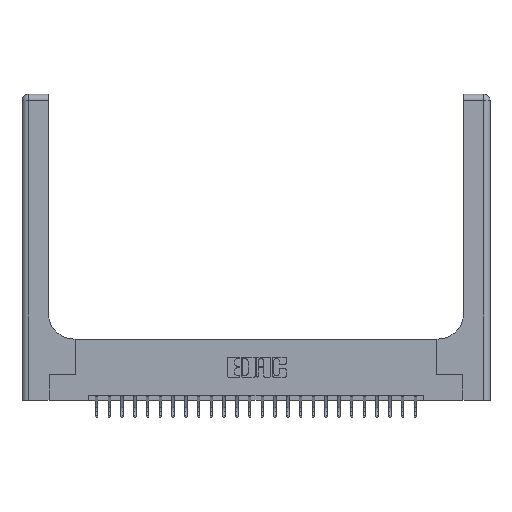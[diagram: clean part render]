
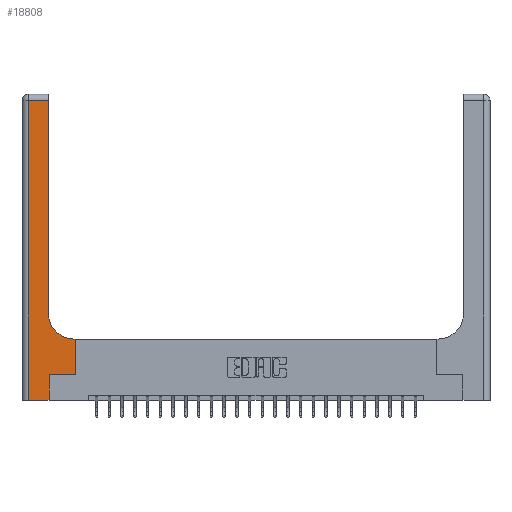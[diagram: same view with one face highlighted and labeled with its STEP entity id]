
A CAD part, top view. The second image highlights one B-rep face of the part: STEP entity #18808.
In plain terms, the highlighted planar face has unit normal (0, 0, 1).
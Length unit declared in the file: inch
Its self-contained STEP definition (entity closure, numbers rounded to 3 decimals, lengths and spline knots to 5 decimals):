
#445 = DIRECTION ( 'NONE',  ( 0., 0., -1. ) ) ;
#733 = CARTESIAN_POINT ( 'NONE',  ( 0.528, 0.25, 0.37 ) ) ;
#1143 = ORIENTED_EDGE ( 'NONE', *, *, #4247, .T. ) ;
#1588 = LINE ( 'NONE', #9330, #21758 ) ;
#1692 = ORIENTED_EDGE ( 'NONE', *, *, #18627, .T. ) ;
#2589 = VERTEX_POINT ( 'NONE', #7430 ) ;
#3351 = VERTEX_POINT ( 'NONE', #3767 ) ;
#3767 = CARTESIAN_POINT ( 'NONE',  ( 0.528, 0.6, 0.37 ) ) ;
#4247 = EDGE_CURVE ( 'NONE', #22149, #6161, #1588, .T. ) ;
#4463 = CARTESIAN_POINT ( 'NONE',  ( 0.51, 0.6, 0.37 ) ) ;
#4517 = CARTESIAN_POINT ( 'NONE',  ( 0.26, 0.6, 0.37 ) ) ;
#4626 = LINE ( 'NONE', #11978, #7910 ) ;
#5216 = ORIENTED_EDGE ( 'NONE', *, *, #20027, .T. ) ;
#5469 = DIRECTION ( 'NONE',  ( 0., 1., 0. ) ) ;
#5540 = VECTOR ( 'NONE', #11737, 39.37008 ) ;
#6161 = VERTEX_POINT ( 'NONE', #20058 ) ;
#6825 = AXIS2_PLACEMENT_3D ( 'NONE', #17399, #445, #23095 ) ;
#7430 = CARTESIAN_POINT ( 'NONE',  ( 0.528, 0.25, 0.37 ) ) ;
#7817 = CARTESIAN_POINT ( 'NONE',  ( 0., 2.94, 0.37 ) ) ;
#7910 = VECTOR ( 'NONE', #10021, 39.37008 ) ;
#8106 = EDGE_CURVE ( 'NONE', #22961, #22149, #9922, .T. ) ;
#8407 = CARTESIAN_POINT ( 'NONE',  ( 0.06, 0., 0.37 ) ) ;
#8592 = VECTOR ( 'NONE', #14252, 39.37008 ) ;
#9330 = CARTESIAN_POINT ( 'NONE',  ( 0.26, 3., 0.37 ) ) ;
#9846 = LINE ( 'NONE', #733, #13367 ) ;
#9863 = CARTESIAN_POINT ( 'NONE',  ( 0.26, 0.85, 0.37 ) ) ;
#9922 = CIRCLE ( 'NONE', #6825, 0.25 ) ;
#10014 = ORIENTED_EDGE ( 'NONE', *, *, #19090, .T. ) ;
#10021 = DIRECTION ( 'NONE',  ( 1., 0., 0. ) ) ;
#10413 = CARTESIAN_POINT ( 'NONE',  ( 0.265, 0.25, 0.37 ) ) ;
#10864 = EDGE_LOOP ( 'NONE', ( #1143, #16876, #10014, #20180, #22399, #1692, #5216, #14372, #19403 ) ) ;
#11556 = VERTEX_POINT ( 'NONE', #20822 ) ;
#11737 = DIRECTION ( 'NONE',  ( 0., 1., 0. ) ) ;
#11818 = DIRECTION ( 'NONE',  ( -1., 0., 0. ) ) ;
#11978 = CARTESIAN_POINT ( 'NONE',  ( 0., 0., 0.37 ) ) ;
#11987 = CARTESIAN_POINT ( 'NONE',  ( 0.06, 2.94, 0.37 ) ) ;
#12107 = LINE ( 'NONE', #17188, #5540 ) ;
#12259 = VECTOR ( 'NONE', #12884, 39.37008 ) ;
#12747 = CARTESIAN_POINT ( 'NONE',  ( 0.06, 3., 0.37 ) ) ;
#12884 = DIRECTION ( 'NONE',  ( 1., 0., 0. ) ) ;
#13367 = VECTOR ( 'NONE', #15728, 39.37008 ) ;
#13483 = VERTEX_POINT ( 'NONE', #11987 ) ;
#13671 = AXIS2_PLACEMENT_3D ( 'NONE', #14956, #14975, #22260 ) ;
#14005 = LINE ( 'NONE', #7817, #24330 ) ;
#14060 = LINE ( 'NONE', #10413, #12259 ) ;
#14252 = DIRECTION ( 'NONE',  ( -1., 0., 0. ) ) ;
#14372 = ORIENTED_EDGE ( 'NONE', *, *, #15848, .T. ) ;
#14433 = EDGE_CURVE ( 'NONE', #6161, #13483, #14005, .T. ) ;
#14675 = DIRECTION ( 'NONE',  ( 0., -1., 0. ) ) ;
#14956 = CARTESIAN_POINT ( 'NONE',  ( 0., 3., 0.37 ) ) ;
#14975 = DIRECTION ( 'NONE',  ( 0., 0., -1. ) ) ;
#15728 = DIRECTION ( 'NONE',  ( 0., 1., 0. ) ) ;
#15821 = VECTOR ( 'NONE', #14675, 39.37008 ) ;
#15848 = EDGE_CURVE ( 'NONE', #3351, #22961, #17748, .T. ) ;
#16415 = FACE_OUTER_BOUND ( 'NONE', #10864, .T. ) ;
#16597 = CARTESIAN_POINT ( 'NONE',  ( 0.265, 0.25, 0.37 ) ) ;
#16876 = ORIENTED_EDGE ( 'NONE', *, *, #14433, .T. ) ;
#17188 = CARTESIAN_POINT ( 'NONE',  ( 0.265, 0., 0.37 ) ) ;
#17399 = CARTESIAN_POINT ( 'NONE',  ( 0.51, 0.85, 0.37 ) ) ;
#17689 = EDGE_CURVE ( 'NONE', #24217, #11556, #4626, .T. ) ;
#17748 = LINE ( 'NONE', #4517, #8592 ) ;
#18627 = EDGE_CURVE ( 'NONE', #20467, #2589, #14060, .T. ) ;
#18808 = ADVANCED_FACE ( 'NONE', ( #16415 ), #21729, .F. ) ;
#19090 = EDGE_CURVE ( 'NONE', #13483, #24217, #23175, .T. ) ;
#19403 = ORIENTED_EDGE ( 'NONE', *, *, #8106, .T. ) ;
#20027 = EDGE_CURVE ( 'NONE', #2589, #3351, #9846, .T. ) ;
#20058 = CARTESIAN_POINT ( 'NONE',  ( 0.26, 2.94, 0.37 ) ) ;
#20180 = ORIENTED_EDGE ( 'NONE', *, *, #17689, .T. ) ;
#20467 = VERTEX_POINT ( 'NONE', #16597 ) ;
#20822 = CARTESIAN_POINT ( 'NONE',  ( 0.265, 0., 0.37 ) ) ;
#21729 = PLANE ( 'NONE',  #13671 ) ;
#21758 = VECTOR ( 'NONE', #5469, 39.37008 ) ;
#21818 = EDGE_CURVE ( 'NONE', #11556, #20467, #12107, .T. ) ;
#22149 = VERTEX_POINT ( 'NONE', #9863 ) ;
#22260 = DIRECTION ( 'NONE',  ( -1., 0., 0. ) ) ;
#22399 = ORIENTED_EDGE ( 'NONE', *, *, #21818, .T. ) ;
#22961 = VERTEX_POINT ( 'NONE', #4463 ) ;
#23095 = DIRECTION ( 'NONE',  ( 1., 0., 0. ) ) ;
#23175 = LINE ( 'NONE', #12747, #15821 ) ;
#24217 = VERTEX_POINT ( 'NONE', #8407 ) ;
#24330 = VECTOR ( 'NONE', #11818, 39.37008 ) ;
